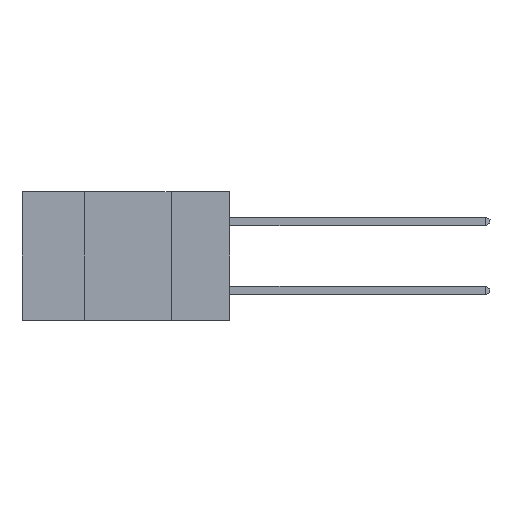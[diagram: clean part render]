
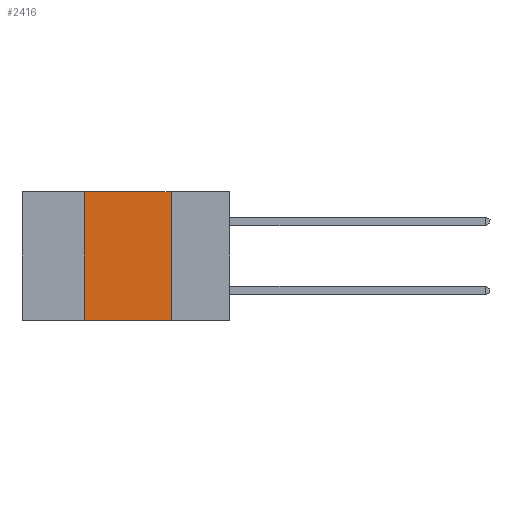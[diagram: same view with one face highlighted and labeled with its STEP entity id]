
A CAD part, left-side view. The second image highlights one B-rep face of the part: STEP entity #2416.
In plain terms, the highlighted planar face has unit normal (-1, 0, 0).
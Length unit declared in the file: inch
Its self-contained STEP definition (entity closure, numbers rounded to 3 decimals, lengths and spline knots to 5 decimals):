
#259 = EDGE_CURVE ( 'NONE', #8596, #5887, #434, .T. ) ;
#314 = DIRECTION ( 'NONE',  ( 0., -1., 0. ) ) ;
#434 = LINE ( 'NONE', #530, #3933 ) ;
#530 = CARTESIAN_POINT ( 'NONE',  ( 0., 0.6, 0. ) ) ;
#1112 = ORIENTED_EDGE ( 'NONE', *, *, #8928, .T. ) ;
#1382 = AXIS2_PLACEMENT_3D ( 'NONE', #2688, #6740, #3455 ) ;
#1581 = DIRECTION ( 'NONE',  ( 0., 0., 1. ) ) ;
#1955 = PLANE ( 'NONE',  #1382 ) ;
#1985 = VECTOR ( 'NONE', #9204, 39.37008 ) ;
#2114 = LINE ( 'NONE', #3560, #5340 ) ;
#2119 = CARTESIAN_POINT ( 'NONE',  ( 0., 0.17, 0. ) ) ;
#2155 = VECTOR ( 'NONE', #1581, 39.37008 ) ;
#2309 = ORIENTED_EDGE ( 'NONE', *, *, #9001, .F. ) ;
#2416 = ADVANCED_FACE ( 'NONE', ( #6540 ), #1955, .F. ) ;
#2688 = CARTESIAN_POINT ( 'NONE',  ( 0., 0.6, 0. ) ) ;
#2937 = LINE ( 'NONE', #5126, #1985 ) ;
#3241 = CARTESIAN_POINT ( 'NONE',  ( 0., 0.42, -0.37 ) ) ;
#3268 = EDGE_CURVE ( 'NONE', #5887, #4374, #2114, .T. ) ;
#3455 = DIRECTION ( 'NONE',  ( 0., 0., -1. ) ) ;
#3560 = CARTESIAN_POINT ( 'NONE',  ( 0., 0.17, -0.37 ) ) ;
#3848 = LINE ( 'NONE', #8473, #2155 ) ;
#3933 = VECTOR ( 'NONE', #314, 39.37008 ) ;
#4374 = VERTEX_POINT ( 'NONE', #5000 ) ;
#4897 = ORIENTED_EDGE ( 'NONE', *, *, #3268, .F. ) ;
#5000 = CARTESIAN_POINT ( 'NONE',  ( 0., 0.17, -0.37 ) ) ;
#5126 = CARTESIAN_POINT ( 'NONE',  ( 0., 0.6, -0.37 ) ) ;
#5340 = VECTOR ( 'NONE', #8283, 39.37008 ) ;
#5578 = ORIENTED_EDGE ( 'NONE', *, *, #259, .F. ) ;
#5887 = VERTEX_POINT ( 'NONE', #2119 ) ;
#6540 = FACE_OUTER_BOUND ( 'NONE', #9308, .T. ) ;
#6740 = DIRECTION ( 'NONE',  ( 1., 0., 0. ) ) ;
#7087 = CARTESIAN_POINT ( 'NONE',  ( 0., 0.42, 0. ) ) ;
#8283 = DIRECTION ( 'NONE',  ( 0., 0., -1. ) ) ;
#8473 = CARTESIAN_POINT ( 'NONE',  ( 0., 0.42, -0.37 ) ) ;
#8596 = VERTEX_POINT ( 'NONE', #7087 ) ;
#8928 = EDGE_CURVE ( 'NONE', #9909, #4374, #2937, .T. ) ;
#9001 = EDGE_CURVE ( 'NONE', #9909, #8596, #3848, .T. ) ;
#9204 = DIRECTION ( 'NONE',  ( 0., -1., 0. ) ) ;
#9308 = EDGE_LOOP ( 'NONE', ( #4897, #5578, #2309, #1112 ) ) ;
#9909 = VERTEX_POINT ( 'NONE', #3241 ) ;
